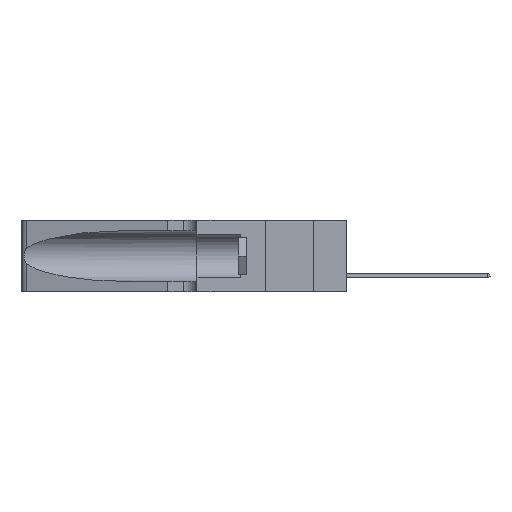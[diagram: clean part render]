
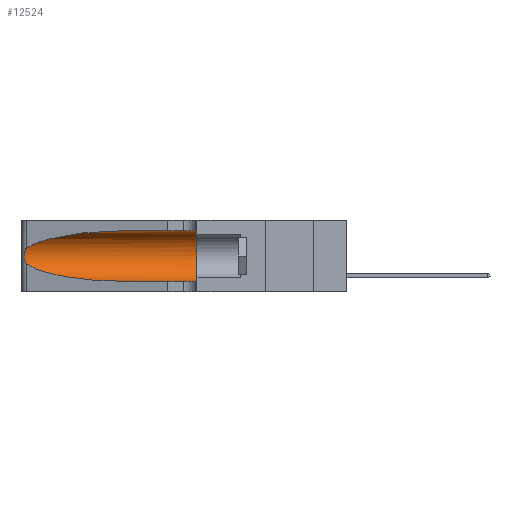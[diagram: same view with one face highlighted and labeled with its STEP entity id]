
A CAD part, left-side view. The second image highlights one B-rep face of the part: STEP entity #12524.
In plain terms, the highlighted cylindrical face has radius 3.308 mm (diameter 6.617 mm), a partial arc.
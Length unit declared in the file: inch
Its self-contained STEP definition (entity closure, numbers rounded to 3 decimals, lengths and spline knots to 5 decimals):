
#819 = CARTESIAN_POINT ( 'NONE',  ( 0.2373, 1.15595, 0.08982 ) ) ;
#1703 = ORIENTED_EDGE ( 'NONE', *, *, #6469, .T. ) ;
#2768 = CARTESIAN_POINT ( 'NONE',  ( 0.18966, 0.96281, 0.31525 ) ) ;
#2874 =( BOUNDED_CURVE ( )  B_SPLINE_CURVE ( 3, ( #26990, #2768, #20434, #11794 ),
 .UNSPECIFIED., .F., .F. ) 
 B_SPLINE_CURVE_WITH_KNOTS ( ( 4, 4 ),
 ( 1.5708, 2.84003 ),
 .UNSPECIFIED. ) 
 CURVE ( )  GEOMETRIC_REPRESENTATION_ITEM ( )  RATIONAL_B_SPLINE_CURVE ( ( 1., 0.87, 0.87, 1. ) ) 
 REPRESENTATION_ITEM ( '' )  );
#3655 = EDGE_CURVE ( 'NONE', #15064, #9545, #23196, .T. ) ;
#4712 = ORIENTED_EDGE ( 'NONE', *, *, #12411, .F. ) ;
#5013 =( BOUNDED_CURVE ( )  B_SPLINE_CURVE ( 3, ( #18294, #819, #27228, #26960 ),
 .UNSPECIFIED., .F., .F. ) 
 B_SPLINE_CURVE_WITH_KNOTS ( ( 4, 4 ),
 ( 3.44316, 4.71239 ),
 .UNSPECIFIED. ) 
 CURVE ( )  GEOMETRIC_REPRESENTATION_ITEM ( )  RATIONAL_B_SPLINE_CURVE ( ( 1., 0.87, 0.87, 1. ) ) 
 REPRESENTATION_ITEM ( '' )  );
#5069 = CIRCLE ( 'NONE', #21064, 0.13025 ) ;
#5425 = EDGE_CURVE ( 'NONE', #13032, #16422, #14397, .T. ) ;
#6469 = EDGE_CURVE ( 'NONE', #26031, #15064, #2874, .T. ) ;
#7340 = CARTESIAN_POINT ( 'NONE',  ( 0.1305, 1.61858, 0.185 ) ) ;
#8079 = CARTESIAN_POINT ( 'NONE',  ( 0.25487, 1.22718, 0.14631 ) ) ;
#8163 = CARTESIAN_POINT ( 'NONE',  ( 0.25555, 1.22994, 0.2215 ) ) ;
#9545 = VERTEX_POINT ( 'NONE', #24722 ) ;
#9596 = DIRECTION ( 'NONE',  ( 0., 0., -1. ) ) ;
#10240 = CARTESIAN_POINT ( 'NONE',  ( 0.25854, 1.2359, 0.20912 ) ) ;
#10513 = CARTESIAN_POINT ( 'NONE',  ( 0.25789, 1.23486, 0.15765 ) ) ;
#10585 = AXIS2_PLACEMENT_3D ( 'NONE', #7340, #24644, #9596 ) ;
#11030 = FACE_OUTER_BOUND ( 'NONE', #23141, .T. ) ;
#11077 = EDGE_CURVE ( 'NONE', #9545, #13032, #5013, .T. ) ;
#11358 = CARTESIAN_POINT ( 'NONE',  ( 0.1305, 0.35, 0.31525 ) ) ;
#11794 = CARTESIAN_POINT ( 'NONE',  ( 0.25487, 1.22718, 0.22369 ) ) ;
#12411 = EDGE_CURVE ( 'NONE', #26031, #24569, #16177, .T. ) ;
#12524 = ADVANCED_FACE ( 'NONE', ( #11030 ), #18235, .F. ) ;
#12549 = CARTESIAN_POINT ( 'NONE',  ( 0.25639, 1.23184, 0.21858 ) ) ;
#12758 = CARTESIAN_POINT ( 'NONE',  ( 0.25856, 1.23593, 0.16098 ) ) ;
#13032 = VERTEX_POINT ( 'NONE', #22865 ) ;
#14378 = ORIENTED_EDGE ( 'NONE', *, *, #5425, .T. ) ;
#14397 = LINE ( 'NONE', #21898, #21609 ) ;
#14678 = DIRECTION ( 'NONE',  ( 0., 0., 1. ) ) ;
#15064 = VERTEX_POINT ( 'NONE', #27803 ) ;
#16177 = LINE ( 'NONE', #23493, #22708 ) ;
#16422 = VERTEX_POINT ( 'NONE', #25389 ) ;
#16493 = CARTESIAN_POINT ( 'NONE',  ( 0.1305, 0.35, 0.185 ) ) ;
#16780 = CARTESIAN_POINT ( 'NONE',  ( 0.26017, 1.23833, 0.17102 ) ) ;
#16874 = CARTESIAN_POINT ( 'NONE',  ( 0.25487, 1.22718, 0.22369 ) ) ;
#16962 = CARTESIAN_POINT ( 'NONE',  ( 0.26018, 1.23835, 0.19895 ) ) ;
#17168 = CARTESIAN_POINT ( 'NONE',  ( 0.26075, 1.23896, 0.178 ) ) ;
#17306 = ORIENTED_EDGE ( 'NONE', *, *, #23988, .F. ) ;
#17572 = ORIENTED_EDGE ( 'NONE', *, *, #3655, .T. ) ;
#17605 = DIRECTION ( 'NONE',  ( 0., -1., 0. ) ) ;
#18235 = CYLINDRICAL_SURFACE ( 'NONE', #10585, 0.13025 ) ;
#18294 = CARTESIAN_POINT ( 'NONE',  ( 0.25487, 1.22718, 0.14631 ) ) ;
#19282 = CARTESIAN_POINT ( 'NONE',  ( 0.25555, 1.22993, 0.14849 ) ) ;
#19854 = CARTESIAN_POINT ( 'NONE',  ( 0.1305, 0.72297, 0.31525 ) ) ;
#20434 = CARTESIAN_POINT ( 'NONE',  ( 0.2373, 1.15595, 0.28018 ) ) ;
#21064 = AXIS2_PLACEMENT_3D ( 'NONE', #16493, #25418, #14678 ) ;
#21191 = CARTESIAN_POINT ( 'NONE',  ( 0.25639, 1.23186, 0.15144 ) ) ;
#21609 = VECTOR ( 'NONE', #17605, 39.37008 ) ;
#21898 = CARTESIAN_POINT ( 'NONE',  ( 0.1305, 1.61858, 0.05475 ) ) ;
#22122 = ORIENTED_EDGE ( 'NONE', *, *, #11077, .T. ) ;
#22708 = VECTOR ( 'NONE', #25714, 39.37008 ) ;
#22865 = CARTESIAN_POINT ( 'NONE',  ( 0.1305, 0.72297, 0.05475 ) ) ;
#23141 = EDGE_LOOP ( 'NONE', ( #1703, #17572, #22122, #14378, #17306, #4712 ) ) ;
#23196 = B_SPLINE_CURVE_WITH_KNOTS ( 'NONE', 3,
 ( #16874, #8163, #12549, #23666, #10240, #16962, #23760, #17168, #16780, #12758, #10513, #21191, #19282, #8079 ),
 .UNSPECIFIED., .F., .F.,
 ( 4, 2, 2, 2, 2, 2, 4 ),
 ( 0., 0.00027, 0.00053, 0.00107, 0.0016, 0.00187, 0.00214 ),
 .UNSPECIFIED. ) ;
#23493 = CARTESIAN_POINT ( 'NONE',  ( 0.1305, 1.61858, 0.31525 ) ) ;
#23666 = CARTESIAN_POINT ( 'NONE',  ( 0.25787, 1.23484, 0.2124 ) ) ;
#23760 = CARTESIAN_POINT ( 'NONE',  ( 0.26075, 1.23896, 0.19203 ) ) ;
#23988 = EDGE_CURVE ( 'NONE', #24569, #16422, #5069, .T. ) ;
#24569 = VERTEX_POINT ( 'NONE', #11358 ) ;
#24644 = DIRECTION ( 'NONE',  ( 0., -1., 0. ) ) ;
#24722 = CARTESIAN_POINT ( 'NONE',  ( 0.25487, 1.22718, 0.14631 ) ) ;
#25389 = CARTESIAN_POINT ( 'NONE',  ( 0.1305, 0.35, 0.05475 ) ) ;
#25418 = DIRECTION ( 'NONE',  ( 0., 1., 0. ) ) ;
#25714 = DIRECTION ( 'NONE',  ( 0., -1., 0. ) ) ;
#26031 = VERTEX_POINT ( 'NONE', #19854 ) ;
#26960 = CARTESIAN_POINT ( 'NONE',  ( 0.1305, 0.72297, 0.05475 ) ) ;
#26990 = CARTESIAN_POINT ( 'NONE',  ( 0.1305, 0.72297, 0.31525 ) ) ;
#27228 = CARTESIAN_POINT ( 'NONE',  ( 0.18966, 0.96281, 0.05475 ) ) ;
#27803 = CARTESIAN_POINT ( 'NONE',  ( 0.25487, 1.22718, 0.22369 ) ) ;
